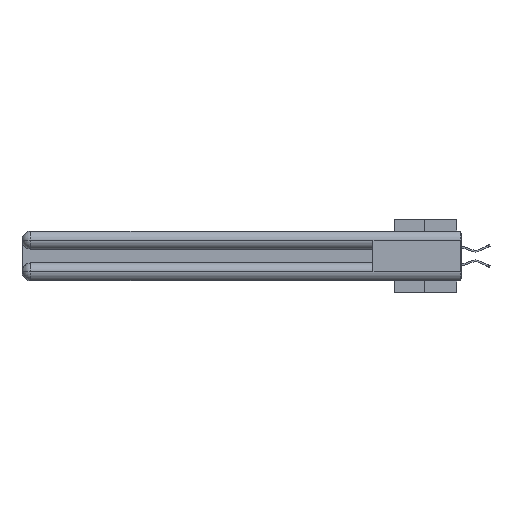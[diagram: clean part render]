
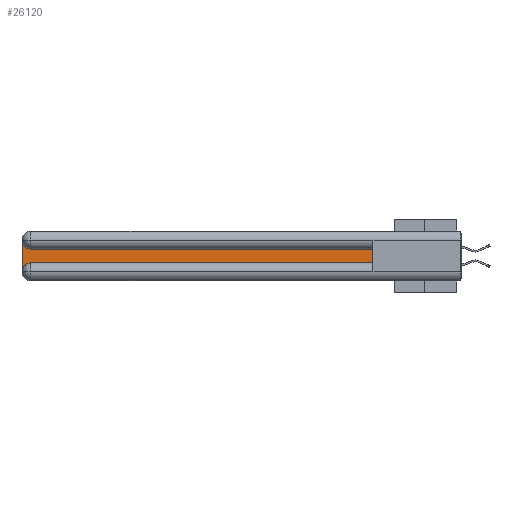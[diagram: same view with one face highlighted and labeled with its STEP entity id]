
A CAD part, left-side view. The second image highlights one B-rep face of the part: STEP entity #26120.
In plain terms, the highlighted planar face has unit normal (-1, 0, 0).
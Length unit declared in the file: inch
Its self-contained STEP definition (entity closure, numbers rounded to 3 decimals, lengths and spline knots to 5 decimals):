
#199 = ORIENTED_EDGE ( 'NONE', *, *, #6588, .T. ) ;
#501 = CARTESIAN_POINT ( 'NONE',  ( 0.075, 0.6, -0.2175 ) ) ;
#821 = LINE ( 'NONE', #31439, #39480 ) ;
#879 = AXIS2_PLACEMENT_3D ( 'NONE', #4758, #27230, #11245 ) ;
#1663 = FACE_OUTER_BOUND ( 'NONE', #40459, .T. ) ;
#1879 = CARTESIAN_POINT ( 'NONE',  ( 0.075, 0.6, -0.2175 ) ) ;
#1881 = ORIENTED_EDGE ( 'NONE', *, *, #35477, .T. ) ;
#2314 = CARTESIAN_POINT ( 'NONE',  ( 0.075, 3., -0.0625 ) ) ;
#2404 = CARTESIAN_POINT ( 'NONE',  ( 0.075, 2.94, -0.0625 ) ) ;
#3256 = CIRCLE ( 'NONE', #33311, 0.06 ) ;
#3451 = CIRCLE ( 'NONE', #879, 0.06 ) ;
#4758 = CARTESIAN_POINT ( 'NONE',  ( 0.075, 2.94, -0.2775 ) ) ;
#5085 = DIRECTION ( 'NONE',  ( 0., 0., -1. ) ) ;
#5865 = LINE ( 'NONE', #34580, #25955 ) ;
#6294 = VECTOR ( 'NONE', #19485, 39.37008 ) ;
#6588 = EDGE_CURVE ( 'NONE', #33395, #34424, #5865, .T. ) ;
#7521 = ORIENTED_EDGE ( 'NONE', *, *, #14799, .T. ) ;
#9285 = VERTEX_POINT ( 'NONE', #36672 ) ;
#11245 = DIRECTION ( 'NONE',  ( 0., 0., -1. ) ) ;
#11717 = DIRECTION ( 'NONE',  ( 1., 0., 0. ) ) ;
#12518 = PLANE ( 'NONE',  #23405 ) ;
#12987 = ORIENTED_EDGE ( 'NONE', *, *, #40568, .T. ) ;
#14799 = EDGE_CURVE ( 'NONE', #39497, #9285, #40227, .T. ) ;
#14861 = LINE ( 'NONE', #501, #6294 ) ;
#15758 = CARTESIAN_POINT ( 'NONE',  ( 0.075, 3., -0.1225 ) ) ;
#19485 = DIRECTION ( 'NONE',  ( 0., -1., 0. ) ) ;
#20178 = CARTESIAN_POINT ( 'NONE',  ( 0.075, 2.94, -0.2175 ) ) ;
#21525 = CARTESIAN_POINT ( 'NONE',  ( 0.075, 0.6, -0.1225 ) ) ;
#21585 = VERTEX_POINT ( 'NONE', #1879 ) ;
#22196 = DIRECTION ( 'NONE',  ( 0., 0., -1. ) ) ;
#23062 = EDGE_CURVE ( 'NONE', #28017, #21585, #14861, .T. ) ;
#23405 = AXIS2_PLACEMENT_3D ( 'NONE', #15758, #32301, #22196 ) ;
#25955 = VECTOR ( 'NONE', #27960, 39.37008 ) ;
#26120 = ADVANCED_FACE ( 'NONE', ( #1663 ), #12518, .F. ) ;
#27230 = DIRECTION ( 'NONE',  ( 1., 0., 0. ) ) ;
#27710 = VECTOR ( 'NONE', #31562, 39.37008 ) ;
#27860 = ORIENTED_EDGE ( 'NONE', *, *, #29727, .T. ) ;
#27960 = DIRECTION ( 'NONE',  ( 0., 1., 0. ) ) ;
#28017 = VERTEX_POINT ( 'NONE', #20178 ) ;
#29727 = EDGE_CURVE ( 'NONE', #21585, #33395, #821, .T. ) ;
#31439 = CARTESIAN_POINT ( 'NONE',  ( 0.075, 0.6, -0.2175 ) ) ;
#31562 = DIRECTION ( 'NONE',  ( 0., 0., -1. ) ) ;
#32301 = DIRECTION ( 'NONE',  ( 1., 0., 0. ) ) ;
#33311 = AXIS2_PLACEMENT_3D ( 'NONE', #2404, #11717, #5085 ) ;
#33395 = VERTEX_POINT ( 'NONE', #21525 ) ;
#34424 = VERTEX_POINT ( 'NONE', #35242 ) ;
#34580 = CARTESIAN_POINT ( 'NONE',  ( 0.075, 0.6, -0.1225 ) ) ;
#34670 = DIRECTION ( 'NONE',  ( 0., 0., 1. ) ) ;
#35242 = CARTESIAN_POINT ( 'NONE',  ( 0.075, 2.94, -0.1225 ) ) ;
#35351 = CARTESIAN_POINT ( 'NONE',  ( 0.075, 3., -0.2175 ) ) ;
#35477 = EDGE_CURVE ( 'NONE', #34424, #39497, #3256, .T. ) ;
#36672 = CARTESIAN_POINT ( 'NONE',  ( 0.075, 3., -0.2775 ) ) ;
#39480 = VECTOR ( 'NONE', #34670, 39.37008 ) ;
#39497 = VERTEX_POINT ( 'NONE', #2314 ) ;
#40227 = LINE ( 'NONE', #35351, #27710 ) ;
#40459 = EDGE_LOOP ( 'NONE', ( #199, #1881, #7521, #12987, #40823, #27860 ) ) ;
#40568 = EDGE_CURVE ( 'NONE', #9285, #28017, #3451, .T. ) ;
#40823 = ORIENTED_EDGE ( 'NONE', *, *, #23062, .T. ) ;
